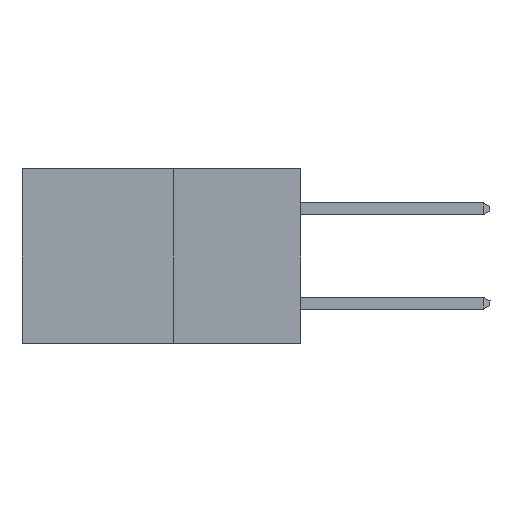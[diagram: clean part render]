
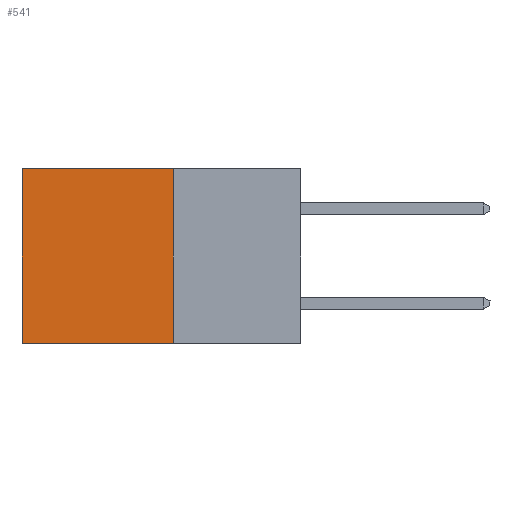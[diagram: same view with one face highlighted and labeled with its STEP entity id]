
A CAD part, left-side view. The second image highlights one B-rep face of the part: STEP entity #541.
In plain terms, the highlighted planar face has unit normal (-1, 0, 0).
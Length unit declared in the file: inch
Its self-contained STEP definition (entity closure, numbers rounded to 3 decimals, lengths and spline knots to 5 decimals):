
#470 = EDGE_CURVE ( 'NONE', #6556, #6404, #4168, .T. ) ;
#541 = ADVANCED_FACE ( 'NONE', ( #8474 ), #6783, .F. ) ;
#1294 = LINE ( 'NONE', #4908, #3238 ) ;
#1848 = DIRECTION ( 'NONE',  ( 0., 0., -1. ) ) ;
#2038 = DIRECTION ( 'NONE',  ( 0., 1., 0. ) ) ;
#2089 = ORIENTED_EDGE ( 'NONE', *, *, #3518, .T. ) ;
#2166 = CARTESIAN_POINT ( 'NONE',  ( 0.277, 0.27, -0.37 ) ) ;
#2194 = CARTESIAN_POINT ( 'NONE',  ( 0.277, 0.27, 0. ) ) ;
#2235 = CARTESIAN_POINT ( 'NONE',  ( 0.277, 0.27, 0. ) ) ;
#2457 = LINE ( 'NONE', #9147, #8106 ) ;
#2475 = VERTEX_POINT ( 'NONE', #6084 ) ;
#2868 = DIRECTION ( 'NONE',  ( 1., 0., 0. ) ) ;
#2991 = ORIENTED_EDGE ( 'NONE', *, *, #6912, .F. ) ;
#3014 = CARTESIAN_POINT ( 'NONE',  ( 0.277, 0.59, 0. ) ) ;
#3238 = VECTOR ( 'NONE', #4855, 39.37008 ) ;
#3457 = ORIENTED_EDGE ( 'NONE', *, *, #5736, .F. ) ;
#3518 = EDGE_CURVE ( 'NONE', #6404, #2475, #1294, .T. ) ;
#3585 = EDGE_LOOP ( 'NONE', ( #2089, #2991, #3457, #8862 ) ) ;
#4168 = LINE ( 'NONE', #2194, #7700 ) ;
#4855 = DIRECTION ( 'NONE',  ( 0., 0., -1. ) ) ;
#4908 = CARTESIAN_POINT ( 'NONE',  ( 0.277, 0.59, -0.37 ) ) ;
#4959 = CARTESIAN_POINT ( 'NONE',  ( 0.277, 0.27, -0.37 ) ) ;
#5736 = EDGE_CURVE ( 'NONE', #6556, #6546, #8864, .T. ) ;
#6084 = CARTESIAN_POINT ( 'NONE',  ( 0.277, 0.59, -0.37 ) ) ;
#6367 = DIRECTION ( 'NONE',  ( 0., 0., -1. ) ) ;
#6404 = VERTEX_POINT ( 'NONE', #3014 ) ;
#6508 = CARTESIAN_POINT ( 'NONE',  ( 0.277, 0.27, -0.37 ) ) ;
#6546 = VERTEX_POINT ( 'NONE', #2166 ) ;
#6556 = VERTEX_POINT ( 'NONE', #2235 ) ;
#6783 = PLANE ( 'NONE',  #8891 ) ;
#6912 = EDGE_CURVE ( 'NONE', #6546, #2475, #2457, .T. ) ;
#6975 = VECTOR ( 'NONE', #6367, 39.37008 ) ;
#7700 = VECTOR ( 'NONE', #2038, 39.37008 ) ;
#8106 = VECTOR ( 'NONE', #9087, 39.37008 ) ;
#8474 = FACE_OUTER_BOUND ( 'NONE', #3585, .T. ) ;
#8862 = ORIENTED_EDGE ( 'NONE', *, *, #470, .T. ) ;
#8864 = LINE ( 'NONE', #6508, #6975 ) ;
#8891 = AXIS2_PLACEMENT_3D ( 'NONE', #4959, #2868, #1848 ) ;
#9087 = DIRECTION ( 'NONE',  ( 0., 1., 0. ) ) ;
#9147 = CARTESIAN_POINT ( 'NONE',  ( 0.277, 0.27, -0.37 ) ) ;
